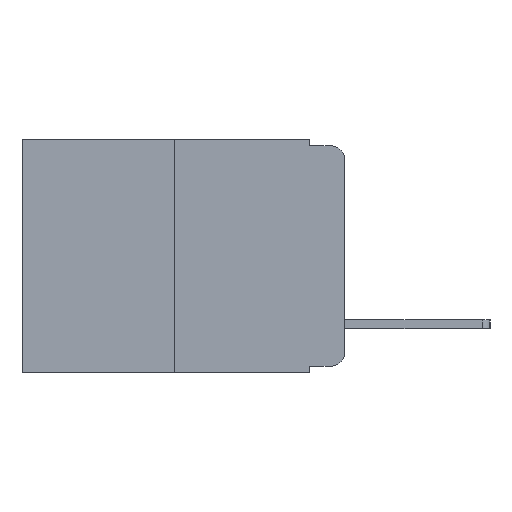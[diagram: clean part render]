
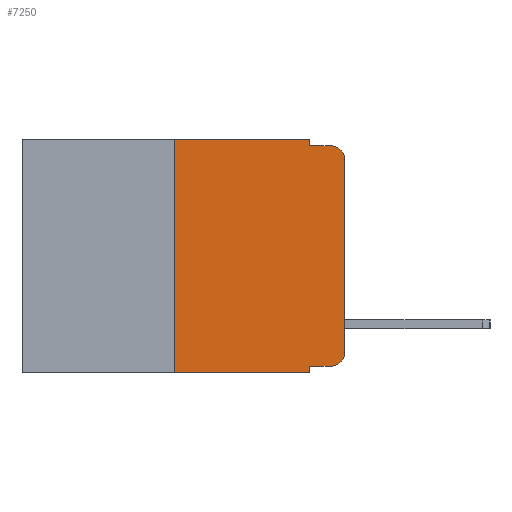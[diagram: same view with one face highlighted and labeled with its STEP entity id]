
A CAD part, left-side view. The second image highlights one B-rep face of the part: STEP entity #7250.
In plain terms, the highlighted planar face has unit normal (-1, 0, 0).
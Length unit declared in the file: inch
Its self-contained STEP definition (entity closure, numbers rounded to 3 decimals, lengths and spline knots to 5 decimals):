
#8 = CARTESIAN_POINT ( 'NONE',  ( 0., 0.051, -0.333 ) ) ;
#230 = EDGE_CURVE ( 'NONE', #8942, #5269, #1047, .T. ) ;
#271 = CARTESIAN_POINT ( 'NONE',  ( 0., 0.051, -0.01 ) ) ;
#665 = CARTESIAN_POINT ( 'NONE',  ( 0., 0.25, 0. ) ) ;
#703 = FACE_OUTER_BOUND ( 'NONE', #9687, .T. ) ;
#1028 = DIRECTION ( 'NONE',  ( 0., -1., 0. ) ) ;
#1047 = LINE ( 'NONE', #5925, #6165 ) ;
#1183 = VERTEX_POINT ( 'NONE', #9550 ) ;
#1486 = DIRECTION ( 'NONE',  ( -1., 0., 0. ) ) ;
#1507 = CARTESIAN_POINT ( 'NONE',  ( 0., 0., -0.313 ) ) ;
#2139 = VECTOR ( 'NONE', #12435, 39.37008 ) ;
#2301 = PLANE ( 'NONE',  #12346 ) ;
#2410 = VERTEX_POINT ( 'NONE', #10834 ) ;
#2492 = AXIS2_PLACEMENT_3D ( 'NONE', #11954, #1486, #8290 ) ;
#2567 = CARTESIAN_POINT ( 'NONE',  ( 0., 0.051, 0. ) ) ;
#2752 = LINE ( 'NONE', #7829, #2139 ) ;
#2766 = VECTOR ( 'NONE', #6400, 39.37008 ) ;
#2822 = EDGE_CURVE ( 'NONE', #1183, #5649, #4455, .T. ) ;
#2834 = CIRCLE ( 'NONE', #11359, 0.02 ) ;
#3074 = EDGE_CURVE ( 'NONE', #6889, #1183, #9378, .T. ) ;
#3076 = VERTEX_POINT ( 'NONE', #4489 ) ;
#3201 = EDGE_CURVE ( 'NONE', #6305, #3076, #8798, .T. ) ;
#3274 = EDGE_CURVE ( 'NONE', #11050, #2410, #2752, .T. ) ;
#3304 = ORIENTED_EDGE ( 'NONE', *, *, #3274, .T. ) ;
#3505 = CIRCLE ( 'NONE', #2492, 0.02 ) ;
#3634 = CARTESIAN_POINT ( 'NONE',  ( 0., 0.473, -0.343 ) ) ;
#4279 = DIRECTION ( 'NONE',  ( 0., 0., -1. ) ) ;
#4455 = LINE ( 'NONE', #271, #7295 ) ;
#4489 = CARTESIAN_POINT ( 'NONE',  ( 0., 0.051, -0.343 ) ) ;
#4504 = EDGE_CURVE ( 'NONE', #7339, #11050, #3505, .T. ) ;
#4619 = DIRECTION ( 'NONE',  ( -1., 0., 0. ) ) ;
#4673 = ORIENTED_EDGE ( 'NONE', *, *, #11051, .F. ) ;
#5255 = LINE ( 'NONE', #3634, #10001 ) ;
#5269 = VERTEX_POINT ( 'NONE', #665 ) ;
#5390 = LINE ( 'NONE', #8311, #2766 ) ;
#5649 = VERTEX_POINT ( 'NONE', #11768 ) ;
#5652 = ORIENTED_EDGE ( 'NONE', *, *, #2822, .F. ) ;
#5739 = CARTESIAN_POINT ( 'NONE',  ( 0., 0.051, -0.333 ) ) ;
#5925 = CARTESIAN_POINT ( 'NONE',  ( 0., 0.25, 0. ) ) ;
#6165 = VECTOR ( 'NONE', #12436, 39.37008 ) ;
#6305 = VERTEX_POINT ( 'NONE', #8 ) ;
#6353 = ORIENTED_EDGE ( 'NONE', *, *, #230, .F. ) ;
#6400 = DIRECTION ( 'NONE',  ( 0., -1., 0. ) ) ;
#6441 = CARTESIAN_POINT ( 'NONE',  ( 0., 0.051, 0. ) ) ;
#6697 = DIRECTION ( 'NONE',  ( 0., -1., 0. ) ) ;
#6749 = EDGE_CURVE ( 'NONE', #2410, #5649, #2834, .T. ) ;
#6784 = ORIENTED_EDGE ( 'NONE', *, *, #6749, .T. ) ;
#6800 = CARTESIAN_POINT ( 'NONE',  ( 0., 0.25, -0.343 ) ) ;
#6889 = VERTEX_POINT ( 'NONE', #10478 ) ;
#7250 = ADVANCED_FACE ( 'NONE', ( #703 ), #2301, .F. ) ;
#7295 = VECTOR ( 'NONE', #1028, 39.37008 ) ;
#7339 = VERTEX_POINT ( 'NONE', #10143 ) ;
#7357 = ORIENTED_EDGE ( 'NONE', *, *, #10429, .T. ) ;
#7495 = DIRECTION ( 'NONE',  ( 0., -1., 0. ) ) ;
#7829 = CARTESIAN_POINT ( 'NONE',  ( 0., 0., 0. ) ) ;
#8281 = ORIENTED_EDGE ( 'NONE', *, *, #3201, .F. ) ;
#8290 = DIRECTION ( 'NONE',  ( 0., 0., -1. ) ) ;
#8311 = CARTESIAN_POINT ( 'NONE',  ( 0., 0.473, 0. ) ) ;
#8332 = ORIENTED_EDGE ( 'NONE', *, *, #3074, .F. ) ;
#8798 = LINE ( 'NONE', #2567, #10389 ) ;
#8942 = VERTEX_POINT ( 'NONE', #6800 ) ;
#8989 = VECTOR ( 'NONE', #6697, 39.37008 ) ;
#9020 = ORIENTED_EDGE ( 'NONE', *, *, #9858, .T. ) ;
#9054 = CARTESIAN_POINT ( 'NONE',  ( 0., 0.473, 0. ) ) ;
#9092 = VECTOR ( 'NONE', #10211, 39.37008 ) ;
#9280 = LINE ( 'NONE', #5739, #8989 ) ;
#9378 = LINE ( 'NONE', #6441, #9092 ) ;
#9550 = CARTESIAN_POINT ( 'NONE',  ( 0., 0.051, -0.01 ) ) ;
#9687 = EDGE_LOOP ( 'NONE', ( #3304, #6784, #5652, #8332, #4673, #6353, #7357, #8281, #9020, #10611 ) ) ;
#9858 = EDGE_CURVE ( 'NONE', #6305, #7339, #9280, .T. ) ;
#9993 = DIRECTION ( 'NONE',  ( 1., 0., 0. ) ) ;
#10001 = VECTOR ( 'NONE', #7495, 39.37008 ) ;
#10143 = CARTESIAN_POINT ( 'NONE',  ( 0., 0.02, -0.333 ) ) ;
#10211 = DIRECTION ( 'NONE',  ( 0., 0., -1. ) ) ;
#10309 = CARTESIAN_POINT ( 'NONE',  ( 0., 0.02, -0.03 ) ) ;
#10389 = VECTOR ( 'NONE', #11058, 39.37008 ) ;
#10429 = EDGE_CURVE ( 'NONE', #8942, #3076, #5255, .T. ) ;
#10478 = CARTESIAN_POINT ( 'NONE',  ( 0., 0.051, 0. ) ) ;
#10611 = ORIENTED_EDGE ( 'NONE', *, *, #4504, .T. ) ;
#10834 = CARTESIAN_POINT ( 'NONE',  ( 0., 0., -0.03 ) ) ;
#11050 = VERTEX_POINT ( 'NONE', #1507 ) ;
#11051 = EDGE_CURVE ( 'NONE', #5269, #6889, #5390, .T. ) ;
#11058 = DIRECTION ( 'NONE',  ( 0., 0., -1. ) ) ;
#11239 = DIRECTION ( 'NONE',  ( 0., 0., -1. ) ) ;
#11359 = AXIS2_PLACEMENT_3D ( 'NONE', #10309, #4619, #11239 ) ;
#11768 = CARTESIAN_POINT ( 'NONE',  ( 0., 0.02, -0.01 ) ) ;
#11954 = CARTESIAN_POINT ( 'NONE',  ( 0., 0.02, -0.313 ) ) ;
#12346 = AXIS2_PLACEMENT_3D ( 'NONE', #9054, #9993, #4279 ) ;
#12435 = DIRECTION ( 'NONE',  ( 0., 0., 1. ) ) ;
#12436 = DIRECTION ( 'NONE',  ( 0., 0., 1. ) ) ;
